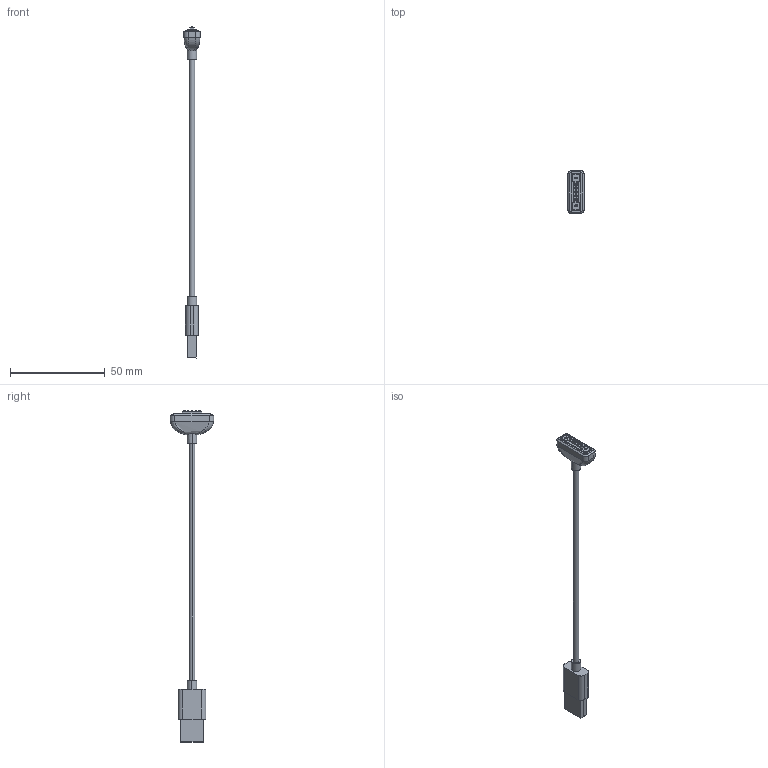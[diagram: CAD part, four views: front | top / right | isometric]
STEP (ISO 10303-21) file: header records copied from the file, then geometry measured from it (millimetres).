
FILE_DESCRIPTION (( 'STEP AP214' ), '1' );
FILE_NAME ('687J0522A51110E.STEP', '2023-05-02T15:15:00', ( '' ), ( '' ), 'SwSTEP 2.0', 'SolidWorks 2020', '' );
FILE_SCHEMA (( 'AUTOMOTIVE_DESIGN' ));
Length unit declared in the file: millimetre
Products named in the file (1): 687J0522A51110E
Bounding box: 8.6 x 22.9 x 175.67 mm (x, y, z)
Volume: 4588.6 mm3; surface area: 4274.4 mm2
Topology: 7 solids, 7 shells, 271 faces, 682 edges, 443 vertices
Faces by surface type: plane 148, cylinder 81, bspline 24, sphere 10, cone 8
Entity records: 12085 total; most frequent: CARTESIAN_POINT 2919, ORIENTED_EDGE 1324, DIRECTION 1278, EDGE_CURVE 662, VERTEX_POINT 433, LINE 426, AXIS2_PLACEMENT_3D 426, VECTOR 426
